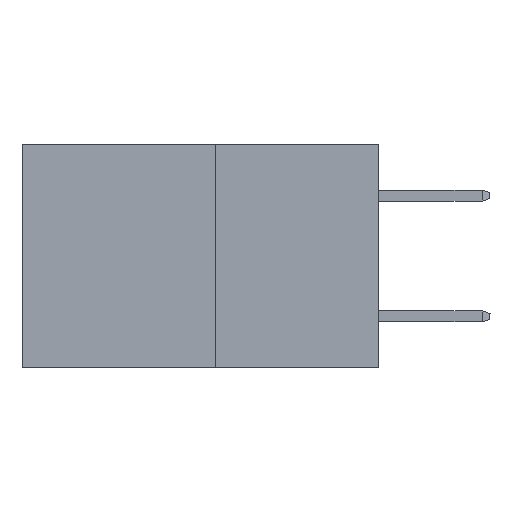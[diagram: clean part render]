
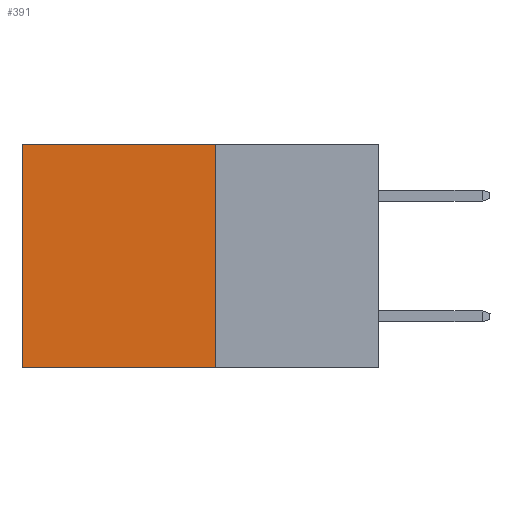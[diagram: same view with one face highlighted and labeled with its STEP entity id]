
A CAD part, left-side view. The second image highlights one B-rep face of the part: STEP entity #391.
In plain terms, the highlighted planar face has unit normal (-1, 0, 0).
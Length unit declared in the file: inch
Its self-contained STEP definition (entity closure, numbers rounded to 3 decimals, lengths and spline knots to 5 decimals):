
#391 = ADVANCED_FACE ( 'NONE', ( #12693 ), #1225, .F. ) ;
#966 = ORIENTED_EDGE ( 'NONE', *, *, #3755, .F. ) ;
#968 = LINE ( 'NONE', #4637, #11631 ) ;
#1139 = LINE ( 'NONE', #4728, #3665 ) ;
#1225 = PLANE ( 'NONE',  #8207 ) ;
#1463 = DIRECTION ( 'NONE',  ( 0., 1., 0. ) ) ;
#1582 = DIRECTION ( 'NONE',  ( 0., 1., 0. ) ) ;
#1807 = VERTEX_POINT ( 'NONE', #12840 ) ;
#1885 = VERTEX_POINT ( 'NONE', #4311 ) ;
#2090 = DIRECTION ( 'NONE',  ( 1., 0., 0. ) ) ;
#2445 = EDGE_CURVE ( 'NONE', #9078, #10110, #1139, .T. ) ;
#2540 = DIRECTION ( 'NONE',  ( 0., 0., -1. ) ) ;
#2746 = LINE ( 'NONE', #5830, #8013 ) ;
#3665 = VECTOR ( 'NONE', #3860, 39.37008 ) ;
#3755 = EDGE_CURVE ( 'NONE', #1807, #1885, #7397, .T. ) ;
#3856 = CARTESIAN_POINT ( 'NONE',  ( 0.277, 0.59, 0. ) ) ;
#3860 = DIRECTION ( 'NONE',  ( 0., 0., -1. ) ) ;
#4311 = CARTESIAN_POINT ( 'NONE',  ( 0.277, 0.27, -0.37 ) ) ;
#4485 = CARTESIAN_POINT ( 'NONE',  ( 0.277, 0.59, -0.37 ) ) ;
#4637 = CARTESIAN_POINT ( 'NONE',  ( 0.277, 0.27, -0.37 ) ) ;
#4728 = CARTESIAN_POINT ( 'NONE',  ( 0.277, 0.59, -0.37 ) ) ;
#5830 = CARTESIAN_POINT ( 'NONE',  ( 0.277, 0.27, 0. ) ) ;
#7051 = ORIENTED_EDGE ( 'NONE', *, *, #2445, .T. ) ;
#7249 = EDGE_LOOP ( 'NONE', ( #7051, #12017, #966, #10896 ) ) ;
#7397 = LINE ( 'NONE', #12951, #10551 ) ;
#8013 = VECTOR ( 'NONE', #1582, 39.37008 ) ;
#8207 = AXIS2_PLACEMENT_3D ( 'NONE', #11867, #2090, #2540 ) ;
#9078 = VERTEX_POINT ( 'NONE', #3856 ) ;
#10110 = VERTEX_POINT ( 'NONE', #4485 ) ;
#10301 = EDGE_CURVE ( 'NONE', #1807, #9078, #2746, .T. ) ;
#10551 = VECTOR ( 'NONE', #12936, 39.37008 ) ;
#10896 = ORIENTED_EDGE ( 'NONE', *, *, #10301, .T. ) ;
#11508 = EDGE_CURVE ( 'NONE', #1885, #10110, #968, .T. ) ;
#11631 = VECTOR ( 'NONE', #1463, 39.37008 ) ;
#11867 = CARTESIAN_POINT ( 'NONE',  ( 0.277, 0.27, -0.37 ) ) ;
#12017 = ORIENTED_EDGE ( 'NONE', *, *, #11508, .F. ) ;
#12693 = FACE_OUTER_BOUND ( 'NONE', #7249, .T. ) ;
#12840 = CARTESIAN_POINT ( 'NONE',  ( 0.277, 0.27, 0. ) ) ;
#12936 = DIRECTION ( 'NONE',  ( 0., 0., -1. ) ) ;
#12951 = CARTESIAN_POINT ( 'NONE',  ( 0.277, 0.27, -0.37 ) ) ;
